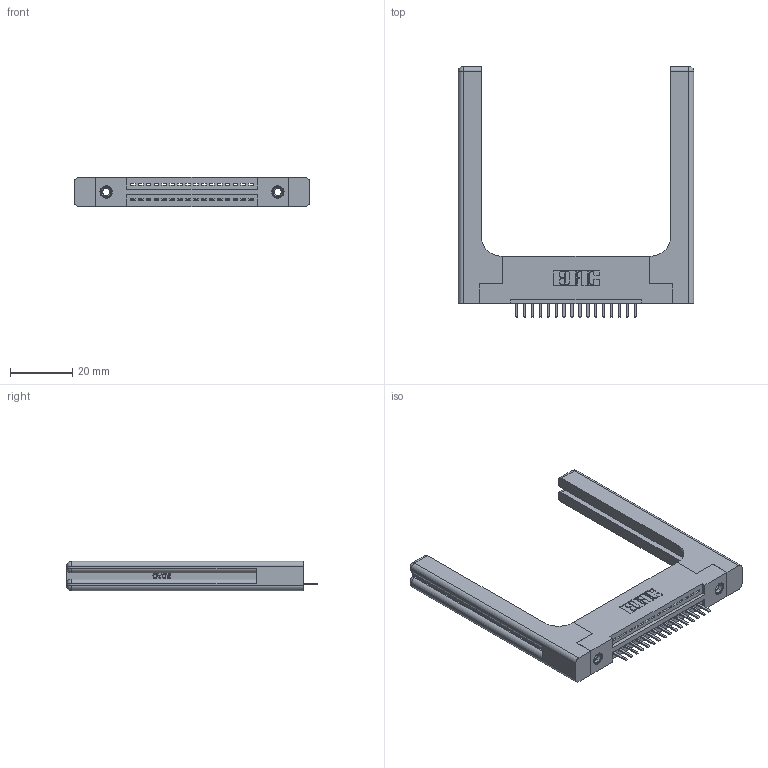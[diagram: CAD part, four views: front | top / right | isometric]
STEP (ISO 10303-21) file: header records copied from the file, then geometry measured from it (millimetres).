
FILE_DESCRIPTION (( 'STEP AP203' ), '1' );
FILE_NAME ('345-016-520-158.STEP', '2019-10-04T13:09:09', ( '' ), ( '' ), 'SwSTEP 2.0', 'SolidWorks 2016', '' );
FILE_SCHEMA (( 'CONFIG_CONTROL_DESIGN' ));
Length unit declared in the file: inch
Products named in the file (5): 345-220-058_345-220-058; 345 Part_Flush Mounting Lugs - 0.156 Dia-TH; 345-292-001_345-293-120; 345-250-001_345-250-001-102; 345-016-520-158
Assembly tree (21 placements, depth 2):
  345-016-520-158
    345 Part_Flush Mounting Lugs - 0.156 Dia-TH
    345-292-001_345-293-120  x16
    345-250-001_345-250-001-102  x2
    345-220-058_345-220-058  x2
Bounding box: 75.67 x 80.64 x 9.4 mm (x, y, z)
Volume: 15432.8 mm3; surface area: 14008.2 mm2
Topology: 21 solids, 21 shells, 1374 faces, 3951 edges, 2570 vertices
Faces by surface type: plane 900, cylinder 414, bspline 36, cone 12, sphere 8, torus 4
Entity records: 20838 total; most frequent: CARTESIAN_POINT 4593, ORIENTED_EDGE 3328, DIRECTION 2984, EDGE_CURVE 1664, VECTOR 1372, LINE 1372, VERTEX_POINT 1098, AXIS2_PLACEMENT_3D 806
